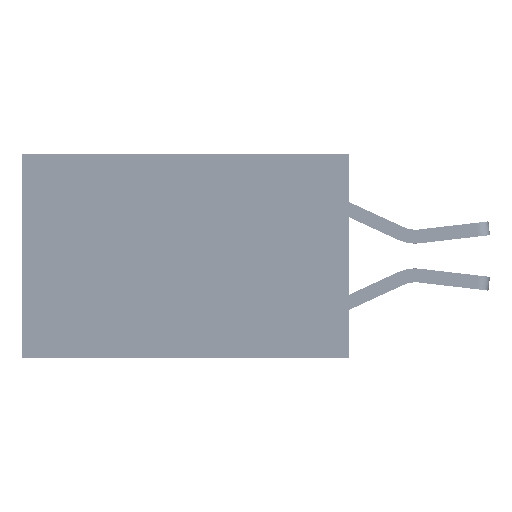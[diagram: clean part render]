
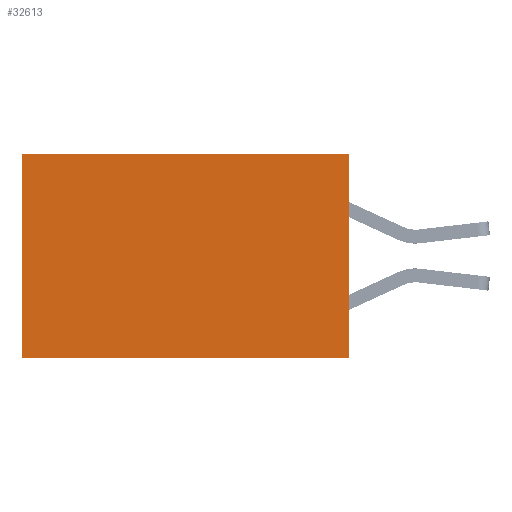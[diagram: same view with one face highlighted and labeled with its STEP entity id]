
A CAD part, left-side view. The second image highlights one B-rep face of the part: STEP entity #32613.
In plain terms, the highlighted planar face has unit normal (-1, 0, 0).
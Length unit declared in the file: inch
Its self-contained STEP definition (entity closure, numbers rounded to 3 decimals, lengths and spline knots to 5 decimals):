
#1560 = EDGE_CURVE ( 'NONE', #31266, #1898, #22827, .T. ) ;
#1572 = EDGE_CURVE ( 'NONE', #4551, #23079, #7943, .T. ) ;
#1898 = VERTEX_POINT ( 'NONE', #33913 ) ;
#4150 = ORIENTED_EDGE ( 'NONE', *, *, #1572, .F. ) ;
#4551 = VERTEX_POINT ( 'NONE', #7123 ) ;
#5059 = VECTOR ( 'NONE', #33929, 39.37008 ) ;
#6253 = EDGE_CURVE ( 'NONE', #1898, #23079, #12967, .T. ) ;
#7123 = CARTESIAN_POINT ( 'NONE',  ( 0.277, 0., -0.37 ) ) ;
#7943 = LINE ( 'NONE', #27105, #21193 ) ;
#9319 = ORIENTED_EDGE ( 'NONE', *, *, #32972, .F. ) ;
#11224 = CARTESIAN_POINT ( 'NONE',  ( 0.277, 0., 0. ) ) ;
#12967 = LINE ( 'NONE', #34146, #5059 ) ;
#13633 = CARTESIAN_POINT ( 'NONE',  ( 0.277, 0., -0.37 ) ) ;
#14927 = VECTOR ( 'NONE', #20116, 39.37008 ) ;
#15997 = CARTESIAN_POINT ( 'NONE',  ( 0.277, 0.59, -0.37 ) ) ;
#16285 = DIRECTION ( 'NONE',  ( 0., 0., -1. ) ) ;
#16476 = CARTESIAN_POINT ( 'NONE',  ( 0.277, 0., 0. ) ) ;
#18864 = EDGE_LOOP ( 'NONE', ( #30470, #4150, #9319, #24465 ) ) ;
#20116 = DIRECTION ( 'NONE',  ( 0., 1., 0. ) ) ;
#21193 = VECTOR ( 'NONE', #32736, 39.37008 ) ;
#21433 = PLANE ( 'NONE',  #27723 ) ;
#22827 = LINE ( 'NONE', #11224, #14927 ) ;
#23079 = VERTEX_POINT ( 'NONE', #15997 ) ;
#24465 = ORIENTED_EDGE ( 'NONE', *, *, #1560, .T. ) ;
#25518 = DIRECTION ( 'NONE',  ( 0., 0., -1. ) ) ;
#26708 = VECTOR ( 'NONE', #25518, 39.37008 ) ;
#27105 = CARTESIAN_POINT ( 'NONE',  ( 0.277, 0., -0.37 ) ) ;
#27723 = AXIS2_PLACEMENT_3D ( 'NONE', #13633, #31968, #16285 ) ;
#30318 = FACE_OUTER_BOUND ( 'NONE', #18864, .T. ) ;
#30470 = ORIENTED_EDGE ( 'NONE', *, *, #6253, .T. ) ;
#30565 = CARTESIAN_POINT ( 'NONE',  ( 0.277, 0., -0.37 ) ) ;
#31266 = VERTEX_POINT ( 'NONE', #16476 ) ;
#31968 = DIRECTION ( 'NONE',  ( 1., 0., 0. ) ) ;
#32613 = ADVANCED_FACE ( 'NONE', ( #30318 ), #21433, .F. ) ;
#32736 = DIRECTION ( 'NONE',  ( 0., 1., 0. ) ) ;
#32972 = EDGE_CURVE ( 'NONE', #31266, #4551, #33569, .T. ) ;
#33569 = LINE ( 'NONE', #30565, #26708 ) ;
#33913 = CARTESIAN_POINT ( 'NONE',  ( 0.277, 0.59, 0. ) ) ;
#33929 = DIRECTION ( 'NONE',  ( 0., 0., -1. ) ) ;
#34146 = CARTESIAN_POINT ( 'NONE',  ( 0.277, 0.59, -0.37 ) ) ;
